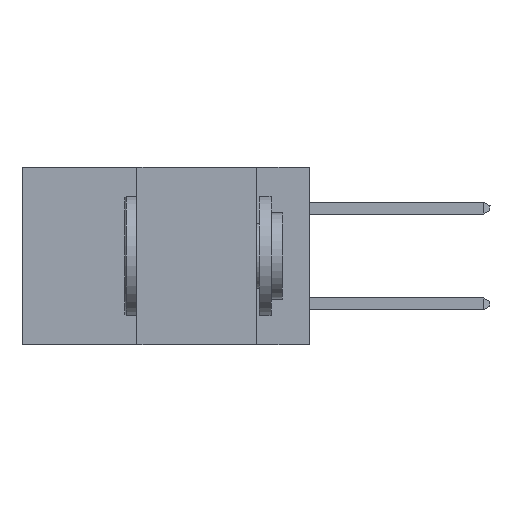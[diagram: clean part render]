
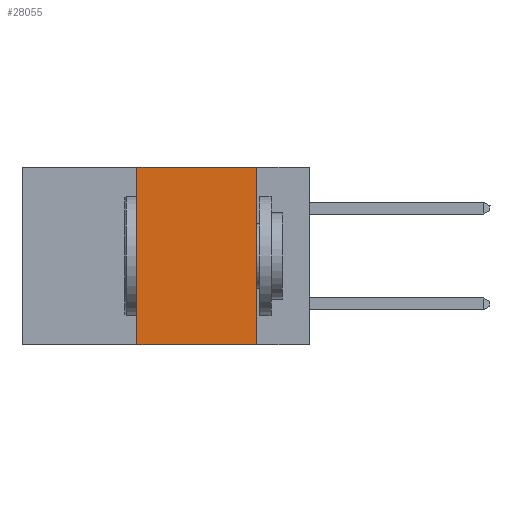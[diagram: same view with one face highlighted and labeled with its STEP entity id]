
A CAD part, left-side view. The second image highlights one B-rep face of the part: STEP entity #28055.
In plain terms, the highlighted planar face has unit normal (-1, 0, 0).
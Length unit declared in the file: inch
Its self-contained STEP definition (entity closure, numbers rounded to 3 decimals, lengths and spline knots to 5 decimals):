
#934 = ORIENTED_EDGE ( 'NONE', *, *, #13982, .F. ) ;
#1071 = CARTESIAN_POINT ( 'NONE',  ( 0., 0.6, -0.37 ) ) ;
#2091 = DIRECTION ( 'NONE',  ( 0., -1., 0. ) ) ;
#5227 = DIRECTION ( 'NONE',  ( 0., 0., -1. ) ) ;
#6193 = VERTEX_POINT ( 'NONE', #33291 ) ;
#10999 = ORIENTED_EDGE ( 'NONE', *, *, #14209, .T. ) ;
#13982 = EDGE_CURVE ( 'NONE', #6193, #44739, #36076, .T. ) ;
#14209 = EDGE_CURVE ( 'NONE', #6193, #18860, #32200, .T. ) ;
#14266 = EDGE_CURVE ( 'NONE', #32344, #18860, #31553, .T. ) ;
#17642 = CARTESIAN_POINT ( 'NONE',  ( 0., 0.6, 0. ) ) ;
#18846 = CARTESIAN_POINT ( 'NONE',  ( 0., 0.11, -0.37 ) ) ;
#18860 = VERTEX_POINT ( 'NONE', #18846 ) ;
#19739 = EDGE_LOOP ( 'NONE', ( #32211, #35447, #934, #10999 ) ) ;
#21159 = EDGE_CURVE ( 'NONE', #44739, #32344, #25980, .T. ) ;
#21212 = DIRECTION ( 'NONE',  ( 0., 0., -1. ) ) ;
#23021 = DIRECTION ( 'NONE',  ( 0., -1., 0. ) ) ;
#24906 = CARTESIAN_POINT ( 'NONE',  ( 0., 0.36, 0. ) ) ;
#25039 = AXIS2_PLACEMENT_3D ( 'NONE', #17642, #42112, #21212 ) ;
#25856 = VECTOR ( 'NONE', #2091, 39.37008 ) ;
#25980 = LINE ( 'NONE', #44747, #25856 ) ;
#26963 = FACE_OUTER_BOUND ( 'NONE', #19739, .T. ) ;
#28055 = ADVANCED_FACE ( 'NONE', ( #26963 ), #38711, .F. ) ;
#31380 = VECTOR ( 'NONE', #5227, 39.37008 ) ;
#31553 = LINE ( 'NONE', #37255, #31380 ) ;
#32200 = LINE ( 'NONE', #1071, #32337 ) ;
#32211 = ORIENTED_EDGE ( 'NONE', *, *, #14266, .F. ) ;
#32337 = VECTOR ( 'NONE', #23021, 39.37008 ) ;
#32344 = VERTEX_POINT ( 'NONE', #37712 ) ;
#33291 = CARTESIAN_POINT ( 'NONE',  ( 0., 0.36, -0.37 ) ) ;
#35447 = ORIENTED_EDGE ( 'NONE', *, *, #21159, .F. ) ;
#35544 = VECTOR ( 'NONE', #35623, 39.37008 ) ;
#35623 = DIRECTION ( 'NONE',  ( 0., 0., 1. ) ) ;
#36076 = LINE ( 'NONE', #45787, #35544 ) ;
#37255 = CARTESIAN_POINT ( 'NONE',  ( 0., 0.11, 0. ) ) ;
#37712 = CARTESIAN_POINT ( 'NONE',  ( 0., 0.11, 0. ) ) ;
#38711 = PLANE ( 'NONE',  #25039 ) ;
#42112 = DIRECTION ( 'NONE',  ( 1., 0., 0. ) ) ;
#44739 = VERTEX_POINT ( 'NONE', #24906 ) ;
#44747 = CARTESIAN_POINT ( 'NONE',  ( 0., 0.6, 0. ) ) ;
#45787 = CARTESIAN_POINT ( 'NONE',  ( 0., 0.36, 0. ) ) ;
